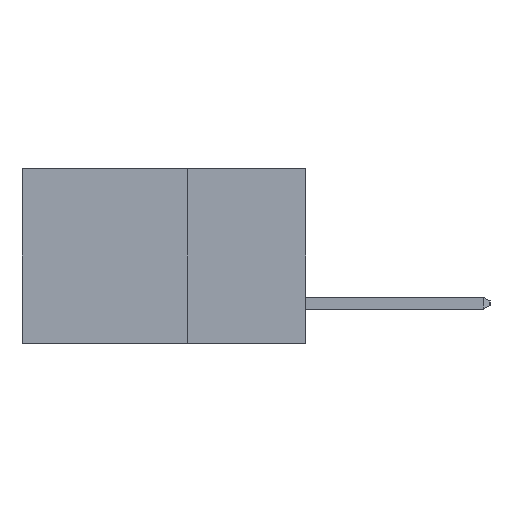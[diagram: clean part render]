
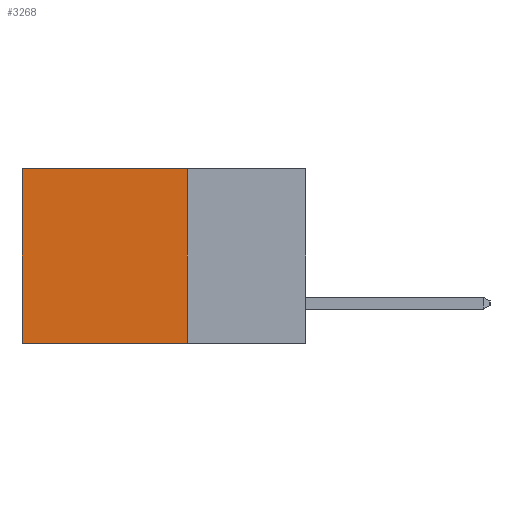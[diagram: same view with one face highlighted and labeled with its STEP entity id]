
A CAD part, left-side view. The second image highlights one B-rep face of the part: STEP entity #3268.
In plain terms, the highlighted planar face has unit normal (-1, 0, 0).
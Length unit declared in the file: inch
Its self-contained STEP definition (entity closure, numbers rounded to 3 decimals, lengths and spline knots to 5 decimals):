
#214 = DIRECTION ( 'NONE',  ( 0., 0., -1. ) ) ;
#1549 = EDGE_CURVE ( 'NONE', #18215, #7550, #12959, .T. ) ;
#1731 = VERTEX_POINT ( 'NONE', #10753 ) ;
#3268 = ADVANCED_FACE ( 'NONE', ( #9678 ), #16763, .F. ) ;
#3399 = EDGE_CURVE ( 'NONE', #7550, #1731, #19276, .T. ) ;
#4531 = ORIENTED_EDGE ( 'NONE', *, *, #3399, .T. ) ;
#5033 = EDGE_LOOP ( 'NONE', ( #4531, #8407, #9126, #15857 ) ) ;
#5277 = EDGE_CURVE ( 'NONE', #15225, #1731, #17359, .T. ) ;
#6991 = DIRECTION ( 'NONE',  ( 0., 1., 0. ) ) ;
#7550 = VERTEX_POINT ( 'NONE', #17692 ) ;
#8287 = VECTOR ( 'NONE', #214, 39.37008 ) ;
#8407 = ORIENTED_EDGE ( 'NONE', *, *, #5277, .F. ) ;
#8568 = VECTOR ( 'NONE', #18265, 39.37008 ) ;
#9126 = ORIENTED_EDGE ( 'NONE', *, *, #13281, .F. ) ;
#9375 = VECTOR ( 'NONE', #6991, 39.37008 ) ;
#9575 = CARTESIAN_POINT ( 'NONE',  ( 0.298, 0.6, 0. ) ) ;
#9678 = FACE_OUTER_BOUND ( 'NONE', #5033, .T. ) ;
#9711 = LINE ( 'NONE', #10534, #17706 ) ;
#10534 = CARTESIAN_POINT ( 'NONE',  ( 0.298, 0.25, 0. ) ) ;
#10753 = CARTESIAN_POINT ( 'NONE',  ( 0.298, 0.6, -0.37 ) ) ;
#12387 = CARTESIAN_POINT ( 'NONE',  ( 0.298, 0.25, -0.37 ) ) ;
#12959 = LINE ( 'NONE', #18426, #8568 ) ;
#13281 = EDGE_CURVE ( 'NONE', #18215, #15225, #9711, .T. ) ;
#14767 = DIRECTION ( 'NONE',  ( 1., 0., 0. ) ) ;
#15210 = AXIS2_PLACEMENT_3D ( 'NONE', #16496, #14767, #17097 ) ;
#15225 = VERTEX_POINT ( 'NONE', #18295 ) ;
#15857 = ORIENTED_EDGE ( 'NONE', *, *, #1549, .T. ) ;
#16496 = CARTESIAN_POINT ( 'NONE',  ( 0.298, 0.25, 0. ) ) ;
#16763 = PLANE ( 'NONE',  #15210 ) ;
#17097 = DIRECTION ( 'NONE',  ( 0., 0., -1. ) ) ;
#17359 = LINE ( 'NONE', #12387, #9375 ) ;
#17667 = CARTESIAN_POINT ( 'NONE',  ( 0.298, 0.25, 0. ) ) ;
#17692 = CARTESIAN_POINT ( 'NONE',  ( 0.298, 0.6, 0. ) ) ;
#17706 = VECTOR ( 'NONE', #19513, 39.37008 ) ;
#18215 = VERTEX_POINT ( 'NONE', #17667 ) ;
#18265 = DIRECTION ( 'NONE',  ( 0., 1., 0. ) ) ;
#18295 = CARTESIAN_POINT ( 'NONE',  ( 0.298, 0.25, -0.37 ) ) ;
#18426 = CARTESIAN_POINT ( 'NONE',  ( 0.298, 0.25, 0. ) ) ;
#19276 = LINE ( 'NONE', #9575, #8287 ) ;
#19513 = DIRECTION ( 'NONE',  ( 0., 0., -1. ) ) ;
